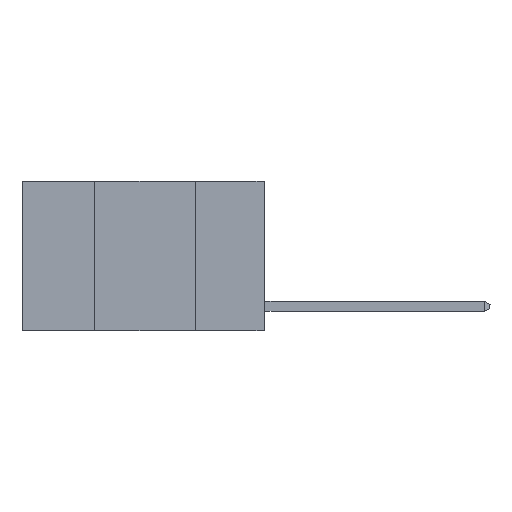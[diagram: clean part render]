
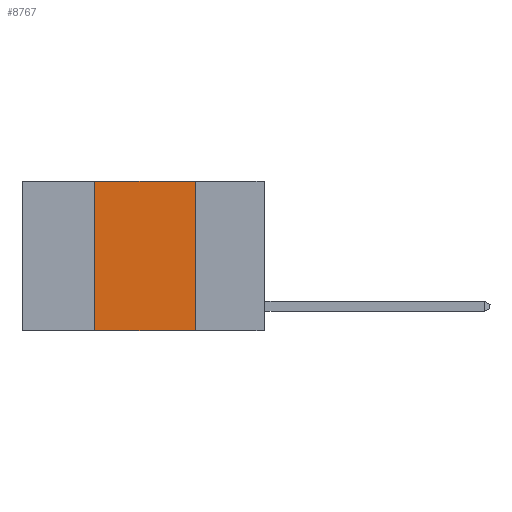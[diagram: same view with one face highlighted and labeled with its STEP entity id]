
A CAD part, left-side view. The second image highlights one B-rep face of the part: STEP entity #8767.
In plain terms, the highlighted planar face has unit normal (-1, 0, 0).
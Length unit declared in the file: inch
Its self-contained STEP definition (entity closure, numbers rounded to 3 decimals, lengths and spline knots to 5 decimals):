
#96 = FACE_OUTER_BOUND ( 'NONE', #12217, .T. ) ;
#977 = CARTESIAN_POINT ( 'NONE',  ( 0., 0.6, 0. ) ) ;
#1112 = CARTESIAN_POINT ( 'NONE',  ( 0., 0.42, 0. ) ) ;
#1122 = LINE ( 'NONE', #7763, #10769 ) ;
#1653 = ORIENTED_EDGE ( 'NONE', *, *, #21089, .T. ) ;
#1926 = CARTESIAN_POINT ( 'NONE',  ( 0., 0.17, -0.37 ) ) ;
#3800 = ORIENTED_EDGE ( 'NONE', *, *, #13573, .F. ) ;
#4286 = EDGE_CURVE ( 'NONE', #15589, #10413, #23680, .T. ) ;
#4448 = VECTOR ( 'NONE', #21020, 39.37008 ) ;
#4894 = DIRECTION ( 'NONE',  ( 1., 0., 0. ) ) ;
#7186 = AXIS2_PLACEMENT_3D ( 'NONE', #977, #4894, #18056 ) ;
#7299 = EDGE_CURVE ( 'NONE', #13258, #15589, #22678, .T. ) ;
#7732 = VECTOR ( 'NONE', #24242, 39.37008 ) ;
#7763 = CARTESIAN_POINT ( 'NONE',  ( 0., 0.42, 0. ) ) ;
#8767 = ADVANCED_FACE ( 'NONE', ( #96 ), #12450, .F. ) ;
#9722 = DIRECTION ( 'NONE',  ( 0., 0., 1. ) ) ;
#9981 = CARTESIAN_POINT ( 'NONE',  ( 0., 0.17, 0. ) ) ;
#10413 = VERTEX_POINT ( 'NONE', #1926 ) ;
#10769 = VECTOR ( 'NONE', #9722, 39.37008 ) ;
#11865 = CARTESIAN_POINT ( 'NONE',  ( 0., 0.42, -0.37 ) ) ;
#12217 = EDGE_LOOP ( 'NONE', ( #15333, #22089, #3800, #1653 ) ) ;
#12323 = VERTEX_POINT ( 'NONE', #11865 ) ;
#12450 = PLANE ( 'NONE',  #7186 ) ;
#13258 = VERTEX_POINT ( 'NONE', #1112 ) ;
#13573 = EDGE_CURVE ( 'NONE', #12323, #13258, #1122, .T. ) ;
#15333 = ORIENTED_EDGE ( 'NONE', *, *, #4286, .F. ) ;
#15589 = VERTEX_POINT ( 'NONE', #16212 ) ;
#16212 = CARTESIAN_POINT ( 'NONE',  ( 0., 0.17, 0. ) ) ;
#18056 = DIRECTION ( 'NONE',  ( 0., 0., -1. ) ) ;
#19124 = CARTESIAN_POINT ( 'NONE',  ( 0., 0.6, -0.37 ) ) ;
#19299 = VECTOR ( 'NONE', #23013, 39.37008 ) ;
#19486 = LINE ( 'NONE', #19124, #4448 ) ;
#21020 = DIRECTION ( 'NONE',  ( 0., -1., 0. ) ) ;
#21089 = EDGE_CURVE ( 'NONE', #12323, #10413, #19486, .T. ) ;
#22089 = ORIENTED_EDGE ( 'NONE', *, *, #7299, .F. ) ;
#22376 = CARTESIAN_POINT ( 'NONE',  ( 0., 0.6, 0. ) ) ;
#22678 = LINE ( 'NONE', #22376, #7732 ) ;
#23013 = DIRECTION ( 'NONE',  ( 0., 0., -1. ) ) ;
#23680 = LINE ( 'NONE', #9981, #19299 ) ;
#24242 = DIRECTION ( 'NONE',  ( 0., -1., 0. ) ) ;
